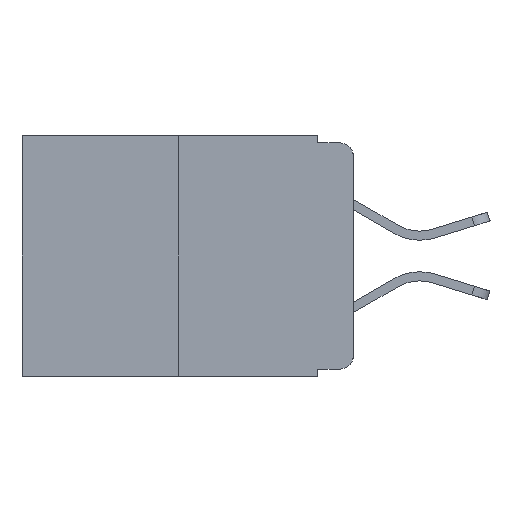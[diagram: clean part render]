
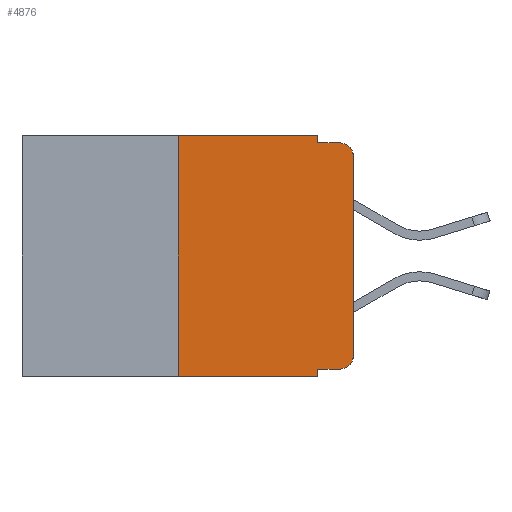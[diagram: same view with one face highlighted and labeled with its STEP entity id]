
A CAD part, left-side view. The second image highlights one B-rep face of the part: STEP entity #4876.
In plain terms, the highlighted planar face has unit normal (-1, 0, 0).
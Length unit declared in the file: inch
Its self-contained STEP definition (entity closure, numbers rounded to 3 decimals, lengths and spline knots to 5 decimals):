
#210 = DIRECTION ( 'NONE',  ( 0., -1., 0. ) ) ;
#521 = CARTESIAN_POINT ( 'NONE',  ( 0., 0.25, 0. ) ) ;
#944 = DIRECTION ( 'NONE',  ( 0., 0., -1. ) ) ;
#1134 = EDGE_CURVE ( 'NONE', #6222, #8472, #20083, .T. ) ;
#1149 = VERTEX_POINT ( 'NONE', #14074 ) ;
#1210 = EDGE_CURVE ( 'NONE', #19320, #19750, #13336, .T. ) ;
#1216 = ORIENTED_EDGE ( 'NONE', *, *, #6517, .F. ) ;
#1896 = VECTOR ( 'NONE', #2007, 39.37008 ) ;
#2007 = DIRECTION ( 'NONE',  ( 0., -1., 0. ) ) ;
#3711 = VECTOR ( 'NONE', #210, 39.37008 ) ;
#3832 = VECTOR ( 'NONE', #9112, 39.37008 ) ;
#3993 = EDGE_CURVE ( 'NONE', #20638, #10997, #18993, .T. ) ;
#4876 = ADVANCED_FACE ( 'NONE', ( #5974 ), #9744, .F. ) ;
#5061 = CARTESIAN_POINT ( 'NONE',  ( 0., 0.25, 0. ) ) ;
#5301 = LINE ( 'NONE', #12142, #25358 ) ;
#5537 = VECTOR ( 'NONE', #944, 39.37008 ) ;
#5701 = EDGE_CURVE ( 'NONE', #17402, #1149, #15280, .T. ) ;
#5974 = FACE_OUTER_BOUND ( 'NONE', #19655, .T. ) ;
#6084 = VECTOR ( 'NONE', #21071, 39.37008 ) ;
#6222 = VERTEX_POINT ( 'NONE', #10237 ) ;
#6423 = DIRECTION ( 'NONE',  ( 0., 0., -1. ) ) ;
#6517 = EDGE_CURVE ( 'NONE', #1149, #6222, #5301, .T. ) ;
#6920 = CARTESIAN_POINT ( 'NONE',  ( 0., 0., -0.03 ) ) ;
#7104 = LINE ( 'NONE', #12782, #5537 ) ;
#7249 = VERTEX_POINT ( 'NONE', #14521 ) ;
#7255 = EDGE_CURVE ( 'NONE', #7249, #10997, #7104, .T. ) ;
#7871 = EDGE_CURVE ( 'NONE', #22158, #19320, #17574, .T. ) ;
#8472 = VERTEX_POINT ( 'NONE', #23217 ) ;
#8550 = ORIENTED_EDGE ( 'NONE', *, *, #3993, .T. ) ;
#9112 = DIRECTION ( 'NONE',  ( 0., -1., 0. ) ) ;
#9744 = PLANE ( 'NONE',  #21775 ) ;
#10237 = CARTESIAN_POINT ( 'NONE',  ( 0., 0.051, -0.01 ) ) ;
#10800 = VECTOR ( 'NONE', #21368, 39.37008 ) ;
#10996 = ORIENTED_EDGE ( 'NONE', *, *, #7255, .F. ) ;
#10997 = VERTEX_POINT ( 'NONE', #23529 ) ;
#11058 = LINE ( 'NONE', #15246, #6084 ) ;
#11529 = ORIENTED_EDGE ( 'NONE', *, *, #7871, .T. ) ;
#11684 = CARTESIAN_POINT ( 'NONE',  ( 0., 0.473, 0. ) ) ;
#11705 = AXIS2_PLACEMENT_3D ( 'NONE', #12616, #24385, #24567 ) ;
#12142 = CARTESIAN_POINT ( 'NONE',  ( 0., 0.051, 0. ) ) ;
#12227 = CARTESIAN_POINT ( 'NONE',  ( 0., 0.051, -0.01 ) ) ;
#12258 = ORIENTED_EDGE ( 'NONE', *, *, #5701, .F. ) ;
#12616 = CARTESIAN_POINT ( 'NONE',  ( 0., 0.02, -0.03 ) ) ;
#12782 = CARTESIAN_POINT ( 'NONE',  ( 0., 0.051, 0. ) ) ;
#13336 = LINE ( 'NONE', #19312, #10800 ) ;
#14074 = CARTESIAN_POINT ( 'NONE',  ( 0., 0.051, 0. ) ) ;
#14521 = CARTESIAN_POINT ( 'NONE',  ( 0., 0.051, -0.333 ) ) ;
#14843 = CARTESIAN_POINT ( 'NONE',  ( 0., 0.02, -0.313 ) ) ;
#14908 = ORIENTED_EDGE ( 'NONE', *, *, #1134, .F. ) ;
#15242 = LINE ( 'NONE', #5061, #18903 ) ;
#15246 = CARTESIAN_POINT ( 'NONE',  ( 0., 0.051, -0.333 ) ) ;
#15280 = LINE ( 'NONE', #17637, #1896 ) ;
#15360 = DIRECTION ( 'NONE',  ( 0., 0., -1. ) ) ;
#15808 = CIRCLE ( 'NONE', #11705, 0.02 ) ;
#17402 = VERTEX_POINT ( 'NONE', #521 ) ;
#17574 = CIRCLE ( 'NONE', #20861, 0.02 ) ;
#17637 = CARTESIAN_POINT ( 'NONE',  ( 0., 0.473, 0. ) ) ;
#17844 = CARTESIAN_POINT ( 'NONE',  ( 0., 0.25, -0.343 ) ) ;
#18462 = EDGE_CURVE ( 'NONE', #19750, #8472, #15808, .T. ) ;
#18903 = VECTOR ( 'NONE', #20754, 39.37008 ) ;
#18993 = LINE ( 'NONE', #22703, #3832 ) ;
#19312 = CARTESIAN_POINT ( 'NONE',  ( 0., 0., 0. ) ) ;
#19320 = VERTEX_POINT ( 'NONE', #19682 ) ;
#19655 = EDGE_LOOP ( 'NONE', ( #24123, #20051, #14908, #1216, #12258, #24226, #8550, #10996, #25037, #11529 ) ) ;
#19682 = CARTESIAN_POINT ( 'NONE',  ( 0., 0., -0.313 ) ) ;
#19750 = VERTEX_POINT ( 'NONE', #6920 ) ;
#19897 = EDGE_CURVE ( 'NONE', #7249, #22158, #11058, .T. ) ;
#20051 = ORIENTED_EDGE ( 'NONE', *, *, #18462, .T. ) ;
#20083 = LINE ( 'NONE', #12227, #3711 ) ;
#20266 = CARTESIAN_POINT ( 'NONE',  ( 0., 0.02, -0.333 ) ) ;
#20638 = VERTEX_POINT ( 'NONE', #17844 ) ;
#20754 = DIRECTION ( 'NONE',  ( 0., 0., 1. ) ) ;
#20861 = AXIS2_PLACEMENT_3D ( 'NONE', #14843, #24523, #24615 ) ;
#21071 = DIRECTION ( 'NONE',  ( 0., -1., 0. ) ) ;
#21368 = DIRECTION ( 'NONE',  ( 0., 0., 1. ) ) ;
#21405 = DIRECTION ( 'NONE',  ( 1., 0., 0. ) ) ;
#21775 = AXIS2_PLACEMENT_3D ( 'NONE', #11684, #21405, #15360 ) ;
#22158 = VERTEX_POINT ( 'NONE', #20266 ) ;
#22703 = CARTESIAN_POINT ( 'NONE',  ( 0., 0.473, -0.343 ) ) ;
#22855 = EDGE_CURVE ( 'NONE', #20638, #17402, #15242, .T. ) ;
#23217 = CARTESIAN_POINT ( 'NONE',  ( 0., 0.02, -0.01 ) ) ;
#23529 = CARTESIAN_POINT ( 'NONE',  ( 0., 0.051, -0.343 ) ) ;
#24123 = ORIENTED_EDGE ( 'NONE', *, *, #1210, .T. ) ;
#24226 = ORIENTED_EDGE ( 'NONE', *, *, #22855, .F. ) ;
#24385 = DIRECTION ( 'NONE',  ( -1., 0., 0. ) ) ;
#24523 = DIRECTION ( 'NONE',  ( -1., 0., 0. ) ) ;
#24567 = DIRECTION ( 'NONE',  ( 0., 0., -1. ) ) ;
#24615 = DIRECTION ( 'NONE',  ( 0., 0., -1. ) ) ;
#25037 = ORIENTED_EDGE ( 'NONE', *, *, #19897, .T. ) ;
#25358 = VECTOR ( 'NONE', #6423, 39.37008 ) ;
